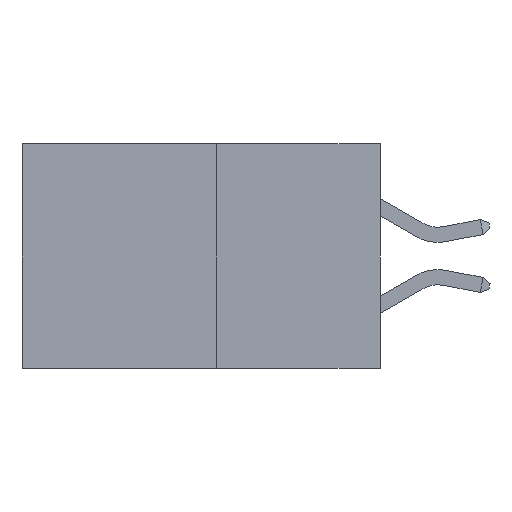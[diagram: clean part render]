
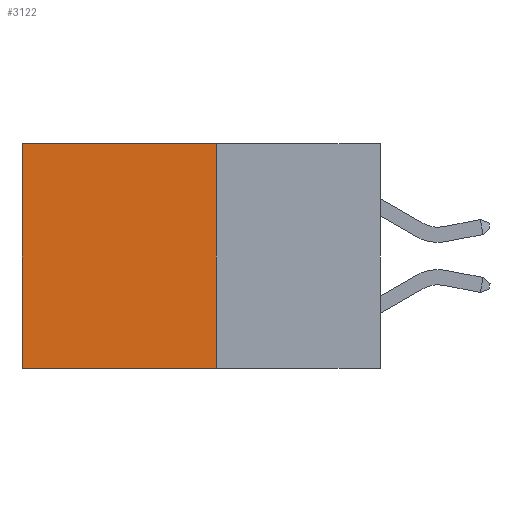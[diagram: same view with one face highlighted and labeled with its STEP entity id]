
A CAD part, left-side view. The second image highlights one B-rep face of the part: STEP entity #3122.
In plain terms, the highlighted planar face has unit normal (-1, 0, 0).
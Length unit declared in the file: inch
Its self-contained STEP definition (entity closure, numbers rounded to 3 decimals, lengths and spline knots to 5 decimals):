
#309 = CARTESIAN_POINT ( 'NONE',  ( 0.277, 0.27, -0.37 ) ) ;
#523 = AXIS2_PLACEMENT_3D ( 'NONE', #2963, #5072, #4908 ) ;
#1839 = EDGE_CURVE ( 'NONE', #17756, #23860, #11262, .T. ) ;
#2010 = CARTESIAN_POINT ( 'NONE',  ( 0.277, 0.27, 0. ) ) ;
#2383 = ORIENTED_EDGE ( 'NONE', *, *, #7598, .F. ) ;
#2963 = CARTESIAN_POINT ( 'NONE',  ( 0.277, 0.27, -0.37 ) ) ;
#3122 = ADVANCED_FACE ( 'NONE', ( #8208 ), #11993, .F. ) ;
#4019 = VERTEX_POINT ( 'NONE', #26580 ) ;
#4908 = DIRECTION ( 'NONE',  ( 0., 0., -1. ) ) ;
#5072 = DIRECTION ( 'NONE',  ( 1., 0., 0. ) ) ;
#6011 = VECTOR ( 'NONE', #14646, 39.37008 ) ;
#6281 = DIRECTION ( 'NONE',  ( 0., 1., 0. ) ) ;
#6355 = CARTESIAN_POINT ( 'NONE',  ( 0.277, 0.27, -0.37 ) ) ;
#6640 = LINE ( 'NONE', #12503, #6011 ) ;
#7598 = EDGE_CURVE ( 'NONE', #23860, #18717, #14156, .T. ) ;
#8208 = FACE_OUTER_BOUND ( 'NONE', #25753, .T. ) ;
#9573 = ORIENTED_EDGE ( 'NONE', *, *, #1839, .F. ) ;
#10472 = DIRECTION ( 'NONE',  ( 0., 0., -1. ) ) ;
#11262 = LINE ( 'NONE', #25477, #25858 ) ;
#11798 = VECTOR ( 'NONE', #22625, 39.37008 ) ;
#11993 = PLANE ( 'NONE',  #523 ) ;
#12503 = CARTESIAN_POINT ( 'NONE',  ( 0.277, 0.27, 0. ) ) ;
#12721 = ORIENTED_EDGE ( 'NONE', *, *, #25611, .T. ) ;
#13242 = ORIENTED_EDGE ( 'NONE', *, *, #21432, .T. ) ;
#14156 = LINE ( 'NONE', #6355, #14806 ) ;
#14280 = CARTESIAN_POINT ( 'NONE',  ( 0.277, 0.59, -0.37 ) ) ;
#14646 = DIRECTION ( 'NONE',  ( 0., 1., 0. ) ) ;
#14806 = VECTOR ( 'NONE', #6281, 39.37008 ) ;
#17756 = VERTEX_POINT ( 'NONE', #2010 ) ;
#18717 = VERTEX_POINT ( 'NONE', #19872 ) ;
#19872 = CARTESIAN_POINT ( 'NONE',  ( 0.277, 0.59, -0.37 ) ) ;
#21432 = EDGE_CURVE ( 'NONE', #4019, #18717, #23552, .T. ) ;
#22625 = DIRECTION ( 'NONE',  ( 0., 0., -1. ) ) ;
#23552 = LINE ( 'NONE', #14280, #11798 ) ;
#23860 = VERTEX_POINT ( 'NONE', #309 ) ;
#25477 = CARTESIAN_POINT ( 'NONE',  ( 0.277, 0.27, -0.37 ) ) ;
#25611 = EDGE_CURVE ( 'NONE', #17756, #4019, #6640, .T. ) ;
#25753 = EDGE_LOOP ( 'NONE', ( #13242, #2383, #9573, #12721 ) ) ;
#25858 = VECTOR ( 'NONE', #10472, 39.37008 ) ;
#26580 = CARTESIAN_POINT ( 'NONE',  ( 0.277, 0.59, 0. ) ) ;
